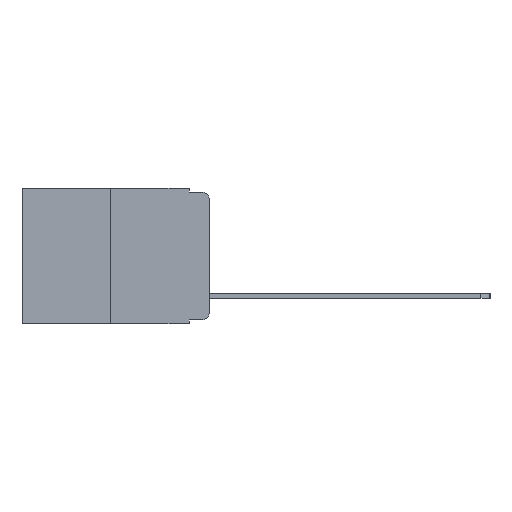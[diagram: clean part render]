
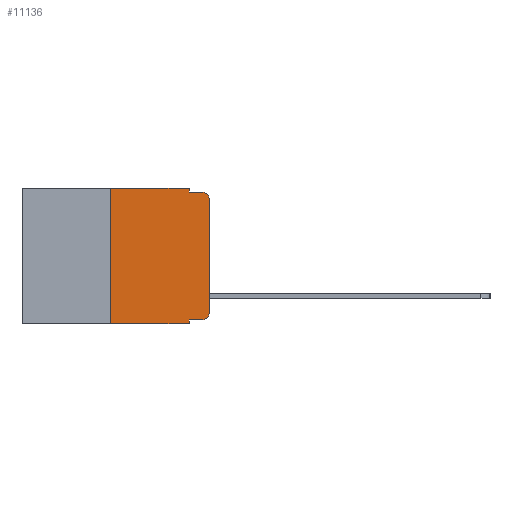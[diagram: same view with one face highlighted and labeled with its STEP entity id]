
A CAD part, left-side view. The second image highlights one B-rep face of the part: STEP entity #11136.
In plain terms, the highlighted planar face has unit normal (-1, 0, 0).
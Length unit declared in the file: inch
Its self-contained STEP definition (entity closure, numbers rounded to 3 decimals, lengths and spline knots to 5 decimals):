
#113 = VERTEX_POINT ( 'NONE', #19337 ) ;
#206 = CIRCLE ( 'NONE', #17130, 0.02 ) ;
#752 = CARTESIAN_POINT ( 'NONE',  ( 0., 0.02, -0.01 ) ) ;
#1483 = CARTESIAN_POINT ( 'NONE',  ( 0., 0.473, -0.343 ) ) ;
#1635 = CARTESIAN_POINT ( 'NONE',  ( 0., 0.25, 0. ) ) ;
#1739 = EDGE_LOOP ( 'NONE', ( #10076, #10639, #6451, #12865, #18725, #15093, #19869, #20398, #12049, #8460 ) ) ;
#2283 = LINE ( 'NONE', #5247, #21288 ) ;
#2701 = VECTOR ( 'NONE', #8926, 39.37008 ) ;
#2877 = LINE ( 'NONE', #10406, #21327 ) ;
#3104 = VECTOR ( 'NONE', #10888, 39.37008 ) ;
#3272 = CARTESIAN_POINT ( 'NONE',  ( 0., 0.02, -0.313 ) ) ;
#3398 = CARTESIAN_POINT ( 'NONE',  ( 0., 0.051, -0.333 ) ) ;
#3669 = LINE ( 'NONE', #1483, #12651 ) ;
#4052 = CARTESIAN_POINT ( 'NONE',  ( 0., 0.051, -0.343 ) ) ;
#4289 = DIRECTION ( 'NONE',  ( -1., 0., 0. ) ) ;
#4938 = LINE ( 'NONE', #21578, #14444 ) ;
#5084 = PLANE ( 'NONE',  #18857 ) ;
#5106 = DIRECTION ( 'NONE',  ( 0., 0., -1. ) ) ;
#5247 = CARTESIAN_POINT ( 'NONE',  ( 0., 0.051, -0.333 ) ) ;
#5294 = VERTEX_POINT ( 'NONE', #752 ) ;
#5499 = DIRECTION ( 'NONE',  ( 0., 0., -1. ) ) ;
#5538 = CARTESIAN_POINT ( 'NONE',  ( 0., 0., -0.313 ) ) ;
#5679 = AXIS2_PLACEMENT_3D ( 'NONE', #3272, #15809, #5106 ) ;
#6451 = ORIENTED_EDGE ( 'NONE', *, *, #18342, .F. ) ;
#7034 = DIRECTION ( 'NONE',  ( 0., 0., -1. ) ) ;
#7393 = CARTESIAN_POINT ( 'NONE',  ( 0., 0.473, 0. ) ) ;
#7687 = FACE_OUTER_BOUND ( 'NONE', #1739, .T. ) ;
#8327 = LINE ( 'NONE', #15970, #21369 ) ;
#8460 = ORIENTED_EDGE ( 'NONE', *, *, #8804, .T. ) ;
#8719 = DIRECTION ( 'NONE',  ( 1., 0., 0. ) ) ;
#8723 = DIRECTION ( 'NONE',  ( 0., 0., 1. ) ) ;
#8804 = EDGE_CURVE ( 'NONE', #9343, #14840, #16494, .T. ) ;
#8926 = DIRECTION ( 'NONE',  ( 0., 0., 1. ) ) ;
#8975 = VERTEX_POINT ( 'NONE', #18159 ) ;
#9173 = DIRECTION ( 'NONE',  ( 0., -1., 0. ) ) ;
#9300 = VERTEX_POINT ( 'NONE', #13822 ) ;
#9343 = VERTEX_POINT ( 'NONE', #13897 ) ;
#10076 = ORIENTED_EDGE ( 'NONE', *, *, #23086, .T. ) ;
#10328 = VERTEX_POINT ( 'NONE', #13542 ) ;
#10406 = CARTESIAN_POINT ( 'NONE',  ( 0., 0., 0. ) ) ;
#10639 = ORIENTED_EDGE ( 'NONE', *, *, #20712, .T. ) ;
#10888 = DIRECTION ( 'NONE',  ( 0., -1., 0. ) ) ;
#10897 = CARTESIAN_POINT ( 'NONE',  ( 0., 0.051, 0. ) ) ;
#11136 = ADVANCED_FACE ( 'NONE', ( #7687 ), #5084, .F. ) ;
#11186 = EDGE_CURVE ( 'NONE', #21436, #9343, #2283, .T. ) ;
#11345 = EDGE_CURVE ( 'NONE', #15198, #10328, #22108, .T. ) ;
#12049 = ORIENTED_EDGE ( 'NONE', *, *, #11186, .T. ) ;
#12240 = CARTESIAN_POINT ( 'NONE',  ( 0., 0.25, 0. ) ) ;
#12651 = VECTOR ( 'NONE', #22970, 39.37008 ) ;
#12865 = ORIENTED_EDGE ( 'NONE', *, *, #17137, .F. ) ;
#13541 = EDGE_CURVE ( 'NONE', #21436, #17822, #16186, .T. ) ;
#13542 = CARTESIAN_POINT ( 'NONE',  ( 0., 0.051, 0. ) ) ;
#13822 = CARTESIAN_POINT ( 'NONE',  ( 0., 0., -0.03 ) ) ;
#13897 = CARTESIAN_POINT ( 'NONE',  ( 0., 0.02, -0.333 ) ) ;
#14444 = VECTOR ( 'NONE', #9173, 39.37008 ) ;
#14740 = EDGE_CURVE ( 'NONE', #8975, #15198, #17550, .T. ) ;
#14840 = VERTEX_POINT ( 'NONE', #5538 ) ;
#14992 = CARTESIAN_POINT ( 'NONE',  ( 0., 0.02, -0.03 ) ) ;
#15093 = ORIENTED_EDGE ( 'NONE', *, *, #14740, .F. ) ;
#15198 = VERTEX_POINT ( 'NONE', #12240 ) ;
#15809 = DIRECTION ( 'NONE',  ( -1., 0., 0. ) ) ;
#15943 = DIRECTION ( 'NONE',  ( 0., -1., 0. ) ) ;
#15970 = CARTESIAN_POINT ( 'NONE',  ( 0., 0.051, 0. ) ) ;
#16186 = LINE ( 'NONE', #10897, #20667 ) ;
#16494 = CIRCLE ( 'NONE', #5679, 0.02 ) ;
#16803 = DIRECTION ( 'NONE',  ( 0., 0., -1. ) ) ;
#17130 = AXIS2_PLACEMENT_3D ( 'NONE', #14992, #4289, #16803 ) ;
#17137 = EDGE_CURVE ( 'NONE', #10328, #113, #8327, .T. ) ;
#17550 = LINE ( 'NONE', #1635, #2701 ) ;
#17822 = VERTEX_POINT ( 'NONE', #4052 ) ;
#18159 = CARTESIAN_POINT ( 'NONE',  ( 0., 0.25, -0.343 ) ) ;
#18342 = EDGE_CURVE ( 'NONE', #113, #5294, #4938, .T. ) ;
#18725 = ORIENTED_EDGE ( 'NONE', *, *, #11345, .F. ) ;
#18857 = AXIS2_PLACEMENT_3D ( 'NONE', #19379, #8719, #21144 ) ;
#19337 = CARTESIAN_POINT ( 'NONE',  ( 0., 0.051, -0.01 ) ) ;
#19379 = CARTESIAN_POINT ( 'NONE',  ( 0., 0.473, 0. ) ) ;
#19869 = ORIENTED_EDGE ( 'NONE', *, *, #21010, .T. ) ;
#20398 = ORIENTED_EDGE ( 'NONE', *, *, #13541, .F. ) ;
#20667 = VECTOR ( 'NONE', #5499, 39.37008 ) ;
#20712 = EDGE_CURVE ( 'NONE', #9300, #5294, #206, .T. ) ;
#21010 = EDGE_CURVE ( 'NONE', #8975, #17822, #3669, .T. ) ;
#21144 = DIRECTION ( 'NONE',  ( 0., 0., -1. ) ) ;
#21288 = VECTOR ( 'NONE', #15943, 39.37008 ) ;
#21327 = VECTOR ( 'NONE', #8723, 39.37008 ) ;
#21369 = VECTOR ( 'NONE', #7034, 39.37008 ) ;
#21436 = VERTEX_POINT ( 'NONE', #3398 ) ;
#21578 = CARTESIAN_POINT ( 'NONE',  ( 0., 0.051, -0.01 ) ) ;
#22108 = LINE ( 'NONE', #7393, #3104 ) ;
#22970 = DIRECTION ( 'NONE',  ( 0., -1., 0. ) ) ;
#23086 = EDGE_CURVE ( 'NONE', #14840, #9300, #2877, .T. ) ;
